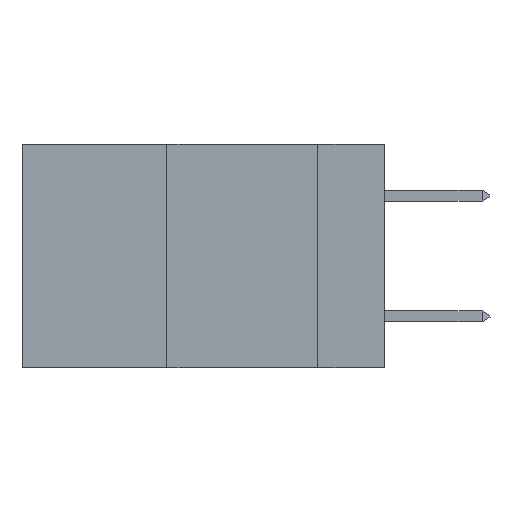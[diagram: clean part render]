
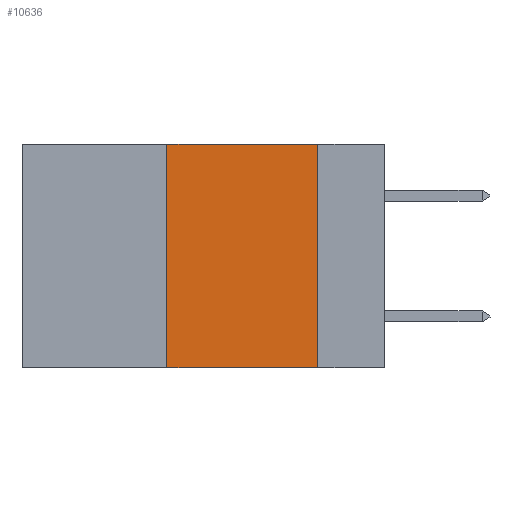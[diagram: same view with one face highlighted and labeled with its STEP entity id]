
A CAD part, left-side view. The second image highlights one B-rep face of the part: STEP entity #10636.
In plain terms, the highlighted planar face has unit normal (-1, 0, 0).
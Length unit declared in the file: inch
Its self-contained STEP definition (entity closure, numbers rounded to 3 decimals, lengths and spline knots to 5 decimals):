
#1764 = CARTESIAN_POINT ( 'NONE',  ( 0., 0.36, -0.37 ) ) ;
#2505 = ORIENTED_EDGE ( 'NONE', *, *, #10700, .T. ) ;
#2609 = VERTEX_POINT ( 'NONE', #2977 ) ;
#2977 = CARTESIAN_POINT ( 'NONE',  ( 0., 0.36, 0. ) ) ;
#3136 = FACE_OUTER_BOUND ( 'NONE', #8057, .T. ) ;
#3286 = ORIENTED_EDGE ( 'NONE', *, *, #3648, .F. ) ;
#3648 = EDGE_CURVE ( 'NONE', #11738, #6449, #19268, .T. ) ;
#4651 = DIRECTION ( 'NONE',  ( 0., -1., 0. ) ) ;
#5691 = CARTESIAN_POINT ( 'NONE',  ( 0., 0.6, 0. ) ) ;
#5849 = DIRECTION ( 'NONE',  ( 0., -1., 0. ) ) ;
#6089 = VECTOR ( 'NONE', #5849, 39.37008 ) ;
#6204 = VECTOR ( 'NONE', #8121, 39.37008 ) ;
#6449 = VERTEX_POINT ( 'NONE', #10426 ) ;
#7390 = DIRECTION ( 'NONE',  ( 1., 0., 0. ) ) ;
#8057 = EDGE_LOOP ( 'NONE', ( #3286, #10556, #8975, #2505 ) ) ;
#8121 = DIRECTION ( 'NONE',  ( 0., 0., -1. ) ) ;
#8975 = ORIENTED_EDGE ( 'NONE', *, *, #16391, .F. ) ;
#9090 = VECTOR ( 'NONE', #21420, 39.37008 ) ;
#9239 = CARTESIAN_POINT ( 'NONE',  ( 0., 0.6, -0.37 ) ) ;
#9336 = AXIS2_PLACEMENT_3D ( 'NONE', #5691, #7390, #19343 ) ;
#9786 = CARTESIAN_POINT ( 'NONE',  ( 0., 0.6, 0. ) ) ;
#10426 = CARTESIAN_POINT ( 'NONE',  ( 0., 0.11, -0.37 ) ) ;
#10556 = ORIENTED_EDGE ( 'NONE', *, *, #20374, .F. ) ;
#10636 = ADVANCED_FACE ( 'NONE', ( #3136 ), #15934, .F. ) ;
#10644 = LINE ( 'NONE', #9239, #6089 ) ;
#10700 = EDGE_CURVE ( 'NONE', #16028, #6449, #10644, .T. ) ;
#11738 = VERTEX_POINT ( 'NONE', #19005 ) ;
#15934 = PLANE ( 'NONE',  #9336 ) ;
#16028 = VERTEX_POINT ( 'NONE', #1764 ) ;
#16391 = EDGE_CURVE ( 'NONE', #16028, #2609, #18117, .T. ) ;
#16595 = VECTOR ( 'NONE', #4651, 39.37008 ) ;
#18117 = LINE ( 'NONE', #19685, #9090 ) ;
#19005 = CARTESIAN_POINT ( 'NONE',  ( 0., 0.11, 0. ) ) ;
#19268 = LINE ( 'NONE', #21696, #6204 ) ;
#19343 = DIRECTION ( 'NONE',  ( 0., 0., -1. ) ) ;
#19685 = CARTESIAN_POINT ( 'NONE',  ( 0., 0.36, 0. ) ) ;
#20374 = EDGE_CURVE ( 'NONE', #2609, #11738, #21089, .T. ) ;
#21089 = LINE ( 'NONE', #9786, #16595 ) ;
#21420 = DIRECTION ( 'NONE',  ( 0., 0., 1. ) ) ;
#21696 = CARTESIAN_POINT ( 'NONE',  ( 0., 0.11, 0. ) ) ;
